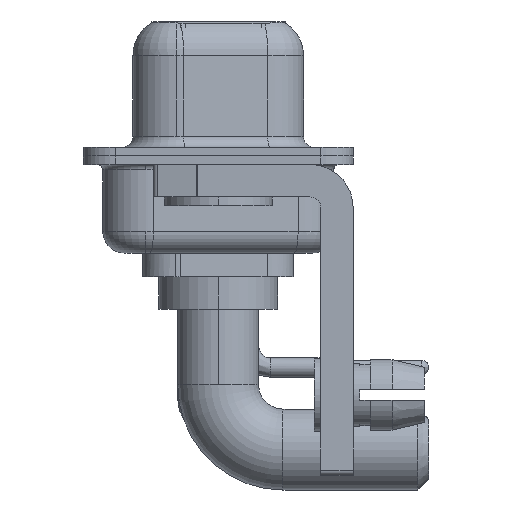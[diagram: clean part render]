
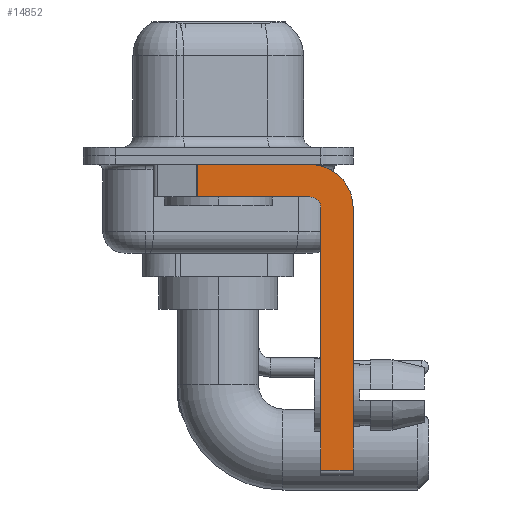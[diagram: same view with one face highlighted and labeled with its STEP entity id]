
A CAD part, left-side view. The second image highlights one B-rep face of the part: STEP entity #14852.
In plain terms, the highlighted planar face has unit normal (-1, 0, 0).
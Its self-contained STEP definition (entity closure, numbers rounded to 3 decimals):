
#846 = DIRECTION ( 'NONE',  ( 0., 0., -1. ) ) ;
#972 = VERTEX_POINT ( 'NONE', #6266 ) ;
#1240 = VERTEX_POINT ( 'NONE', #12542 ) ;
#1606 = EDGE_CURVE ( 'NONE', #11034, #972, #15386, .T. ) ;
#1998 = CARTESIAN_POINT ( 'NONE',  ( -2.9, -6.25, -14.55 ) ) ;
#2122 = CARTESIAN_POINT ( 'NONE',  ( -2.9, -4.25, -14.55 ) ) ;
#2143 = VECTOR ( 'NONE', #19101, 1000. ) ;
#2374 = CARTESIAN_POINT ( 'NONE',  ( -2.9, -4.25, -2.4 ) ) ;
#2743 = VERTEX_POINT ( 'NONE', #20752 ) ;
#3953 = DIRECTION ( 'NONE',  ( 0., -1., 0. ) ) ;
#4031 = DIRECTION ( 'NONE',  ( 0., -1., 0. ) ) ;
#4120 = ORIENTED_EDGE ( 'NONE', *, *, #6292, .T. ) ;
#4334 = VECTOR ( 'NONE', #10029, 1000. ) ;
#4724 = VECTOR ( 'NONE', #10132, 1000. ) ;
#5249 = VERTEX_POINT ( 'NONE', #7995 ) ;
#5253 = CARTESIAN_POINT ( 'NONE',  ( -2.9, -4.25, -0.4 ) ) ;
#5668 = LINE ( 'NONE', #2122, #15456 ) ;
#5772 = PLANE ( 'NONE',  #14463 ) ;
#5904 = EDGE_CURVE ( 'NONE', #5249, #2743, #22260, .T. ) ;
#5999 = CARTESIAN_POINT ( 'NONE',  ( -2.9, -4.25, -2.4 ) ) ;
#6266 = CARTESIAN_POINT ( 'NONE',  ( -2.9, 0.978, -1.9 ) ) ;
#6292 = EDGE_CURVE ( 'NONE', #1240, #972, #8484, .T. ) ;
#6352 = CARTESIAN_POINT ( 'NONE',  ( -2.9, -4.25, -1.9 ) ) ;
#6736 = ORIENTED_EDGE ( 'NONE', *, *, #19572, .T. ) ;
#7428 = ORIENTED_EDGE ( 'NONE', *, *, #5904, .F. ) ;
#7995 = CARTESIAN_POINT ( 'NONE',  ( -2.9, -4.75, -14.55 ) ) ;
#8484 = LINE ( 'NONE', #19218, #2143 ) ;
#8512 = VERTEX_POINT ( 'NONE', #19918 ) ;
#9154 = CIRCLE ( 'NONE', #16435, 0.5 ) ;
#9398 = EDGE_LOOP ( 'NONE', ( #13969, #4120, #21712, #16125, #7428, #6736, #11428, #12920 ) ) ;
#9511 = VECTOR ( 'NONE', #4031, 1000. ) ;
#9914 = DIRECTION ( 'NONE',  ( 0., 1., 0. ) ) ;
#10029 = DIRECTION ( 'NONE',  ( 0., 0., 1. ) ) ;
#10132 = DIRECTION ( 'NONE',  ( 0., 0., -1. ) ) ;
#11016 = CARTESIAN_POINT ( 'NONE',  ( -2.9, -4.25, -2.4 ) ) ;
#11034 = VERTEX_POINT ( 'NONE', #16941 ) ;
#11428 = ORIENTED_EDGE ( 'NONE', *, *, #16396, .F. ) ;
#12072 = CARTESIAN_POINT ( 'NONE',  ( -2.9, -4.75, -14.8 ) ) ;
#12303 = EDGE_CURVE ( 'NONE', #2743, #11034, #9154, .T. ) ;
#12542 = CARTESIAN_POINT ( 'NONE',  ( -2.9, 0.978, -0.4 ) ) ;
#12920 = ORIENTED_EDGE ( 'NONE', *, *, #22212, .F. ) ;
#13709 = VERTEX_POINT ( 'NONE', #1998 ) ;
#13969 = ORIENTED_EDGE ( 'NONE', *, *, #15368, .F. ) ;
#14463 = AXIS2_PLACEMENT_3D ( 'NONE', #5999, #14919, #846 ) ;
#14613 = DIRECTION ( 'NONE',  ( 0., 0., -1. ) ) ;
#14810 = FACE_OUTER_BOUND ( 'NONE', #9398, .T. ) ;
#14852 = ADVANCED_FACE ( 'NONE', ( #14810 ), #5772, .F. ) ;
#14919 = DIRECTION ( 'NONE',  ( 1., 0., 0. ) ) ;
#15368 = EDGE_CURVE ( 'NONE', #1240, #20368, #21773, .T. ) ;
#15386 = LINE ( 'NONE', #6352, #21202 ) ;
#15456 = VECTOR ( 'NONE', #3953, 1000. ) ;
#16125 = ORIENTED_EDGE ( 'NONE', *, *, #12303, .F. ) ;
#16336 = DIRECTION ( 'NONE',  ( 1., 0., 0. ) ) ;
#16396 = EDGE_CURVE ( 'NONE', #8512, #13709, #21379, .T. ) ;
#16435 = AXIS2_PLACEMENT_3D ( 'NONE', #11016, #19699, #17648 ) ;
#16941 = CARTESIAN_POINT ( 'NONE',  ( -2.9, -4.25, -1.9 ) ) ;
#17648 = DIRECTION ( 'NONE',  ( 0., 0., 1. ) ) ;
#19101 = DIRECTION ( 'NONE',  ( 0., 0., -1. ) ) ;
#19218 = CARTESIAN_POINT ( 'NONE',  ( -2.9, 0.978, -1.9 ) ) ;
#19480 = CIRCLE ( 'NONE', #19852, 2. ) ;
#19572 = EDGE_CURVE ( 'NONE', #5249, #13709, #5668, .T. ) ;
#19652 = CARTESIAN_POINT ( 'NONE',  ( -2.9, -6.25, -2.4 ) ) ;
#19699 = DIRECTION ( 'NONE',  ( -1., 0., 0. ) ) ;
#19709 = CARTESIAN_POINT ( 'NONE',  ( -2.9, 3., -0.4 ) ) ;
#19852 = AXIS2_PLACEMENT_3D ( 'NONE', #2374, #16336, #14613 ) ;
#19918 = CARTESIAN_POINT ( 'NONE',  ( -2.9, -6.25, -2.4 ) ) ;
#20368 = VERTEX_POINT ( 'NONE', #5253 ) ;
#20752 = CARTESIAN_POINT ( 'NONE',  ( -2.9, -4.75, -2.4 ) ) ;
#21202 = VECTOR ( 'NONE', #9914, 1000. ) ;
#21379 = LINE ( 'NONE', #19652, #4724 ) ;
#21712 = ORIENTED_EDGE ( 'NONE', *, *, #1606, .F. ) ;
#21773 = LINE ( 'NONE', #19709, #9511 ) ;
#22212 = EDGE_CURVE ( 'NONE', #20368, #8512, #19480, .T. ) ;
#22260 = LINE ( 'NONE', #12072, #4334 ) ;
